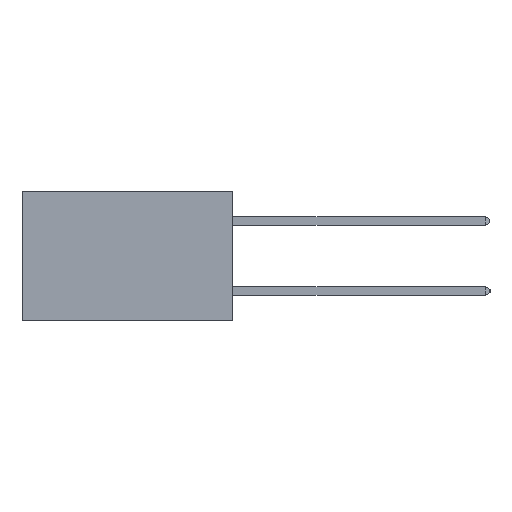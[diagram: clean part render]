
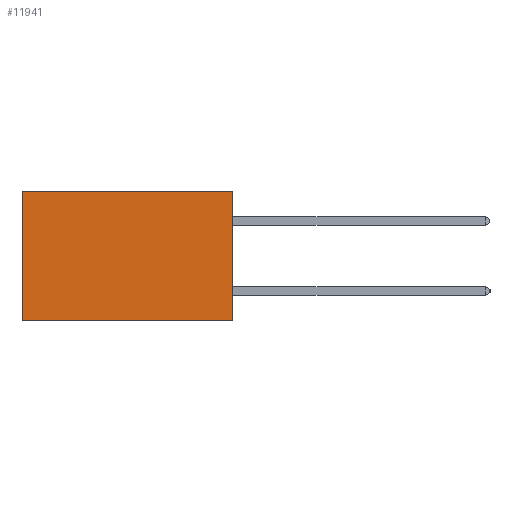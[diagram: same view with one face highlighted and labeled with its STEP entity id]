
A CAD part, left-side view. The second image highlights one B-rep face of the part: STEP entity #11941.
In plain terms, the highlighted planar face has unit normal (-1, 0, 0).
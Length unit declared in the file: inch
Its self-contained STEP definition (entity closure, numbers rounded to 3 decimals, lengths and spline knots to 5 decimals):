
#1307 = PLANE ( 'NONE',  #26354 ) ;
#1683 = VERTEX_POINT ( 'NONE', #17370 ) ;
#2941 = LINE ( 'NONE', #16585, #30827 ) ;
#3017 = CARTESIAN_POINT ( 'NONE',  ( 0.2875, 0., 0. ) ) ;
#3046 = EDGE_LOOP ( 'NONE', ( #4427, #7186, #14870, #13069 ) ) ;
#4159 = LINE ( 'NONE', #26508, #11903 ) ;
#4427 = ORIENTED_EDGE ( 'NONE', *, *, #33020, .T. ) ;
#5646 = EDGE_CURVE ( 'NONE', #21028, #1683, #2941, .T. ) ;
#6598 = DIRECTION ( 'NONE',  ( 0., 1., 0. ) ) ;
#6657 = VERTEX_POINT ( 'NONE', #18752 ) ;
#7186 = ORIENTED_EDGE ( 'NONE', *, *, #13972, .F. ) ;
#8732 = DIRECTION ( 'NONE',  ( 0., 1., 0. ) ) ;
#9868 = CARTESIAN_POINT ( 'NONE',  ( 0.2875, 0., 0. ) ) ;
#10368 = CARTESIAN_POINT ( 'NONE',  ( 0.2875, 0., 0. ) ) ;
#11412 = CARTESIAN_POINT ( 'NONE',  ( 0.2875, 0., -0.37 ) ) ;
#11903 = VECTOR ( 'NONE', #15247, 39.37008 ) ;
#11941 = ADVANCED_FACE ( 'NONE', ( #15827 ), #1307, .F. ) ;
#13069 = ORIENTED_EDGE ( 'NONE', *, *, #5646, .T. ) ;
#13972 = EDGE_CURVE ( 'NONE', #14679, #6657, #14804, .T. ) ;
#14679 = VERTEX_POINT ( 'NONE', #11412 ) ;
#14804 = LINE ( 'NONE', #18058, #29960 ) ;
#14870 = ORIENTED_EDGE ( 'NONE', *, *, #15137, .F. ) ;
#15137 = EDGE_CURVE ( 'NONE', #21028, #14679, #20448, .T. ) ;
#15247 = DIRECTION ( 'NONE',  ( 0., 0., -1. ) ) ;
#15474 = DIRECTION ( 'NONE',  ( 1., 0., 0. ) ) ;
#15827 = FACE_OUTER_BOUND ( 'NONE', #3046, .T. ) ;
#16585 = CARTESIAN_POINT ( 'NONE',  ( 0.2875, 0., 0. ) ) ;
#17370 = CARTESIAN_POINT ( 'NONE',  ( 0.2875, 0.6, 0. ) ) ;
#17712 = DIRECTION ( 'NONE',  ( 0., 0., -1. ) ) ;
#18058 = CARTESIAN_POINT ( 'NONE',  ( 0.2875, 0., -0.37 ) ) ;
#18752 = CARTESIAN_POINT ( 'NONE',  ( 0.2875, 0.6, -0.37 ) ) ;
#20448 = LINE ( 'NONE', #9868, #28279 ) ;
#21028 = VERTEX_POINT ( 'NONE', #3017 ) ;
#26354 = AXIS2_PLACEMENT_3D ( 'NONE', #10368, #15474, #34724 ) ;
#26508 = CARTESIAN_POINT ( 'NONE',  ( 0.2875, 0.6, 0. ) ) ;
#28279 = VECTOR ( 'NONE', #17712, 39.37008 ) ;
#29960 = VECTOR ( 'NONE', #6598, 39.37008 ) ;
#30827 = VECTOR ( 'NONE', #8732, 39.37008 ) ;
#33020 = EDGE_CURVE ( 'NONE', #1683, #6657, #4159, .T. ) ;
#34724 = DIRECTION ( 'NONE',  ( 0., 0., -1. ) ) ;
